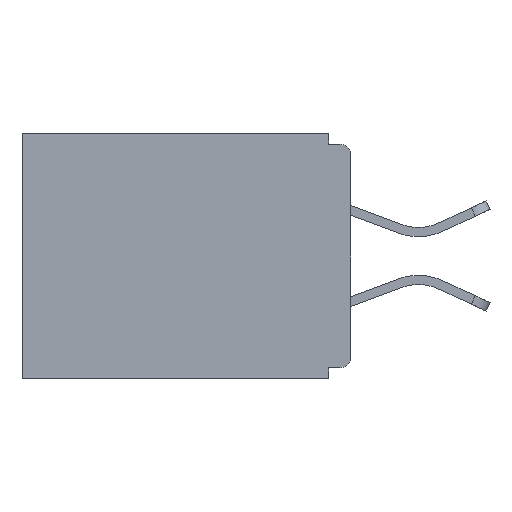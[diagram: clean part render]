
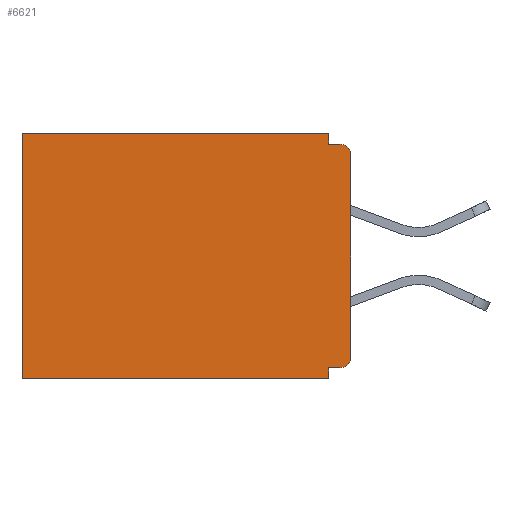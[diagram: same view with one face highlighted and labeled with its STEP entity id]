
A CAD part, left-side view. The second image highlights one B-rep face of the part: STEP entity #6621.
In plain terms, the highlighted planar face has unit normal (-1, 0, 0).
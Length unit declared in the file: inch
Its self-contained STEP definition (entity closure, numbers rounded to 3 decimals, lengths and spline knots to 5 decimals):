
#36 = CARTESIAN_POINT ( 'NONE',  ( 0.298, 0.46, 0. ) ) ;
#389 = DIRECTION ( 'NONE',  ( 0., 1., 0. ) ) ;
#482 = VECTOR ( 'NONE', #15260, 39.37008 ) ;
#735 = CARTESIAN_POINT ( 'NONE',  ( 0.298, 0.031, -0.328 ) ) ;
#790 = EDGE_LOOP ( 'NONE', ( #12121, #7602, #19326, #8416, #18238, #15352, #17871, #4709, #19369, #8725 ) ) ;
#1035 = CARTESIAN_POINT ( 'NONE',  ( 0.298, 0.015, -0.328 ) ) ;
#1416 = LINE ( 'NONE', #13409, #18210 ) ;
#2031 = DIRECTION ( 'NONE',  ( 0., 0., -1. ) ) ;
#2370 = AXIS2_PLACEMENT_3D ( 'NONE', #11413, #3604, #2031 ) ;
#2977 = VECTOR ( 'NONE', #389, 39.37008 ) ;
#3393 = DIRECTION ( 'NONE',  ( 0., 1., 0. ) ) ;
#3604 = DIRECTION ( 'NONE',  ( -1., 0., 0. ) ) ;
#3664 = VERTEX_POINT ( 'NONE', #10121 ) ;
#3778 = DIRECTION ( 'NONE',  ( 0., -1., 0. ) ) ;
#4017 = CARTESIAN_POINT ( 'NONE',  ( 0.298, 0.015, -0.03 ) ) ;
#4083 = DIRECTION ( 'NONE',  ( 0., 1., 0. ) ) ;
#4208 = CARTESIAN_POINT ( 'NONE',  ( 0.298, 0., -0.015 ) ) ;
#4424 = VECTOR ( 'NONE', #12897, 39.37008 ) ;
#4709 = ORIENTED_EDGE ( 'NONE', *, *, #6543, .F. ) ;
#4964 = LINE ( 'NONE', #16884, #11077 ) ;
#5231 = LINE ( 'NONE', #36, #14338 ) ;
#5273 = EDGE_CURVE ( 'NONE', #12497, #8542, #16645, .T. ) ;
#5344 = DIRECTION ( 'NONE',  ( 0., 0., -1. ) ) ;
#5452 = CARTESIAN_POINT ( 'NONE',  ( 0.298, 0.031, -0.343 ) ) ;
#5465 = DIRECTION ( 'NONE',  ( -1., 0., 0. ) ) ;
#5798 = EDGE_CURVE ( 'NONE', #8108, #18751, #5231, .T. ) ;
#6543 = EDGE_CURVE ( 'NONE', #7546, #11272, #7181, .T. ) ;
#6621 = ADVANCED_FACE ( 'NONE', ( #17318 ), #16402, .F. ) ;
#6651 = LINE ( 'NONE', #11458, #482 ) ;
#6793 = CARTESIAN_POINT ( 'NONE',  ( 0.298, 0.46, 0. ) ) ;
#6983 = CARTESIAN_POINT ( 'NONE',  ( 0.298, 0.015, -0.015 ) ) ;
#7181 = LINE ( 'NONE', #19297, #2977 ) ;
#7339 = DIRECTION ( 'NONE',  ( 0., 0., -1. ) ) ;
#7546 = VERTEX_POINT ( 'NONE', #1035 ) ;
#7602 = ORIENTED_EDGE ( 'NONE', *, *, #16450, .F. ) ;
#7612 = LINE ( 'NONE', #8069, #8100 ) ;
#7888 = AXIS2_PLACEMENT_3D ( 'NONE', #15061, #18255, #5344 ) ;
#8069 = CARTESIAN_POINT ( 'NONE',  ( 0.298, 0., -0.343 ) ) ;
#8100 = VECTOR ( 'NONE', #3393, 39.37008 ) ;
#8108 = VERTEX_POINT ( 'NONE', #6793 ) ;
#8416 = ORIENTED_EDGE ( 'NONE', *, *, #19966, .T. ) ;
#8542 = VERTEX_POINT ( 'NONE', #6983 ) ;
#8725 = ORIENTED_EDGE ( 'NONE', *, *, #13558, .F. ) ;
#9715 = VECTOR ( 'NONE', #3778, 39.37008 ) ;
#10121 = CARTESIAN_POINT ( 'NONE',  ( 0.298, 0., -0.313 ) ) ;
#10436 = VERTEX_POINT ( 'NONE', #5452 ) ;
#10545 = CIRCLE ( 'NONE', #2370, 0.015 ) ;
#11077 = VECTOR ( 'NONE', #7339, 39.37008 ) ;
#11272 = VERTEX_POINT ( 'NONE', #735 ) ;
#11367 = CARTESIAN_POINT ( 'NONE',  ( 0.298, 0.031, -0.343 ) ) ;
#11413 = CARTESIAN_POINT ( 'NONE',  ( 0.298, 0.015, -0.313 ) ) ;
#11458 = CARTESIAN_POINT ( 'NONE',  ( 0.298, 0.031, -0.343 ) ) ;
#11784 = LINE ( 'NONE', #11367, #4424 ) ;
#12121 = ORIENTED_EDGE ( 'NONE', *, *, #5273, .T. ) ;
#12456 = LINE ( 'NONE', #4208, #9715 ) ;
#12497 = VERTEX_POINT ( 'NONE', #19486 ) ;
#12897 = DIRECTION ( 'NONE',  ( 0., 0., -1. ) ) ;
#13376 = CARTESIAN_POINT ( 'NONE',  ( 0.298, 0.031, 0. ) ) ;
#13409 = CARTESIAN_POINT ( 'NONE',  ( 0.298, 0., 0. ) ) ;
#13558 = EDGE_CURVE ( 'NONE', #12497, #3664, #4964, .T. ) ;
#14338 = VECTOR ( 'NONE', #19055, 39.37008 ) ;
#14642 = EDGE_CURVE ( 'NONE', #19413, #18873, #6651, .T. ) ;
#15024 = EDGE_CURVE ( 'NONE', #10436, #18751, #7612, .T. ) ;
#15061 = CARTESIAN_POINT ( 'NONE',  ( 0.298, 0., 0. ) ) ;
#15260 = DIRECTION ( 'NONE',  ( 0., 0., -1. ) ) ;
#15352 = ORIENTED_EDGE ( 'NONE', *, *, #15024, .F. ) ;
#16402 = PLANE ( 'NONE',  #7888 ) ;
#16450 = EDGE_CURVE ( 'NONE', #18873, #8542, #12456, .T. ) ;
#16592 = DIRECTION ( 'NONE',  ( 0., 0., -1. ) ) ;
#16645 = CIRCLE ( 'NONE', #17807, 0.015 ) ;
#16884 = CARTESIAN_POINT ( 'NONE',  ( 0.298, 0., 0. ) ) ;
#17318 = FACE_OUTER_BOUND ( 'NONE', #790, .T. ) ;
#17807 = AXIS2_PLACEMENT_3D ( 'NONE', #4017, #5465, #16592 ) ;
#17871 = ORIENTED_EDGE ( 'NONE', *, *, #18492, .F. ) ;
#17987 = EDGE_CURVE ( 'NONE', #7546, #3664, #10545, .T. ) ;
#18210 = VECTOR ( 'NONE', #4083, 39.37008 ) ;
#18238 = ORIENTED_EDGE ( 'NONE', *, *, #5798, .T. ) ;
#18255 = DIRECTION ( 'NONE',  ( 1., 0., 0. ) ) ;
#18492 = EDGE_CURVE ( 'NONE', #11272, #10436, #11784, .T. ) ;
#18602 = CARTESIAN_POINT ( 'NONE',  ( 0.298, 0.46, -0.343 ) ) ;
#18751 = VERTEX_POINT ( 'NONE', #18602 ) ;
#18873 = VERTEX_POINT ( 'NONE', #20102 ) ;
#19055 = DIRECTION ( 'NONE',  ( 0., 0., -1. ) ) ;
#19297 = CARTESIAN_POINT ( 'NONE',  ( 0.298, 0., -0.328 ) ) ;
#19326 = ORIENTED_EDGE ( 'NONE', *, *, #14642, .F. ) ;
#19369 = ORIENTED_EDGE ( 'NONE', *, *, #17987, .T. ) ;
#19413 = VERTEX_POINT ( 'NONE', #13376 ) ;
#19486 = CARTESIAN_POINT ( 'NONE',  ( 0.298, 0., -0.03 ) ) ;
#19966 = EDGE_CURVE ( 'NONE', #19413, #8108, #1416, .T. ) ;
#20102 = CARTESIAN_POINT ( 'NONE',  ( 0.298, 0.031, -0.015 ) ) ;
